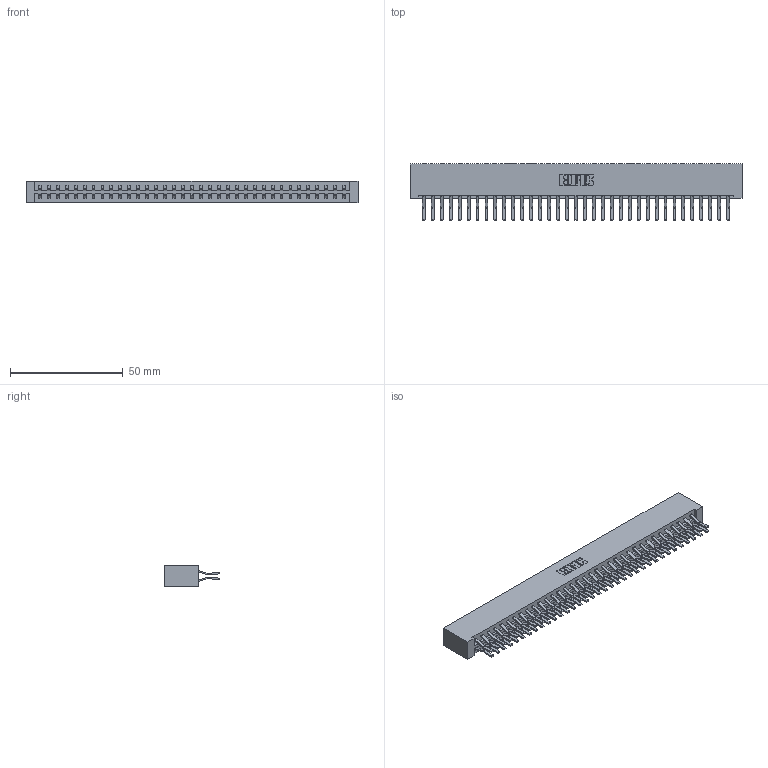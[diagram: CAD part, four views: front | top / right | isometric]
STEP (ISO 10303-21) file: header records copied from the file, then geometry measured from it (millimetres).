
FILE_DESCRIPTION (( 'STEP AP203' ), '1' );
FILE_NAME ('333-070-560-201.STEP', '2018-08-04T15:43:45', ( '' ), ( '' ), 'SwSTEP 2.0', 'SolidWorks 2016', '' );
FILE_SCHEMA (( 'CONFIG_CONTROL_DESIGN' ));
Length unit declared in the file: inch
Products named in the file (3): 333-070-560-201; 333 Part_Lugless; 345-292-001_560 Tail
Assembly tree (71 placements, depth 2):
  333-070-560-201
    333 Part_Lugless
    345-292-001_560 Tail  x70
Bounding box: 146.94 x 24.78 x 9.4 mm (x, y, z)
Volume: 16027.2 mm3; surface area: 20206.2 mm2
Topology: 71 solids, 71 shells, 3886 faces, 11557 edges, 7610 vertices
Faces by surface type: plane 2586, cylinder 1300
Entity records: 23233 total; most frequent: CARTESIAN_POINT 3858, ORIENTED_EDGE 3794, DIRECTION 3305, EDGE_CURVE 1897, LINE 1773, VECTOR 1773, VERTEX_POINT 1262, AXIS2_PLACEMENT_3D 766
